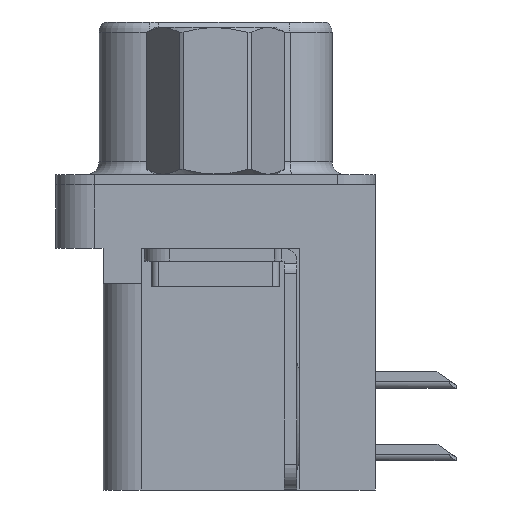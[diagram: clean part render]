
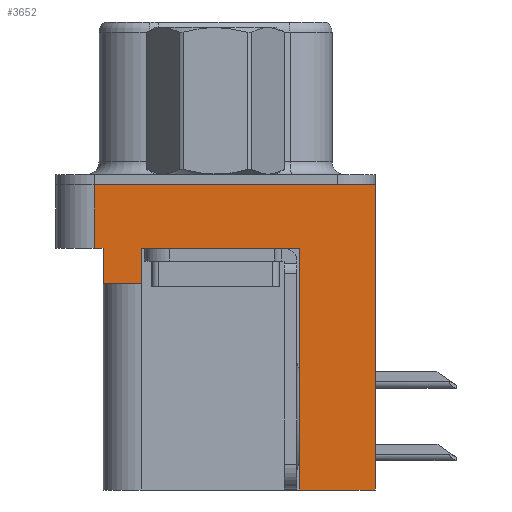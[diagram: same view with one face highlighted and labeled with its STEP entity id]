
A CAD part, left-side view. The second image highlights one B-rep face of the part: STEP entity #3652.
In plain terms, the highlighted planar face has unit normal (-1, 0, 0).
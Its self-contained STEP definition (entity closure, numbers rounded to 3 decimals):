
#145 = VECTOR ( 'NONE', #4610, 1000. ) ;
#225 = EDGE_CURVE ( 'NONE', #10620, #2807, #2601, .T. ) ;
#402 = EDGE_CURVE ( 'NONE', #2580, #18324, #10570, .T. ) ;
#906 = DIRECTION ( 'NONE',  ( 0., -1., 0. ) ) ;
#934 = ORIENTED_EDGE ( 'NONE', *, *, #18183, .T. ) ;
#1684 = DIRECTION ( 'NONE',  ( 0., 1., 0. ) ) ;
#2019 = CARTESIAN_POINT ( 'NONE',  ( -2.91, 2.895, -3.9 ) ) ;
#2459 = ORIENTED_EDGE ( 'NONE', *, *, #12348, .F. ) ;
#2580 = VERTEX_POINT ( 'NONE', #21307 ) ;
#2601 = LINE ( 'NONE', #19234, #7861 ) ;
#2807 = VERTEX_POINT ( 'NONE', #4406 ) ;
#2844 = CARTESIAN_POINT ( 'NONE',  ( -2.91, 2.895, -3.9 ) ) ;
#3044 = CARTESIAN_POINT ( 'NONE',  ( -2.91, 2.895, -2.5 ) ) ;
#3150 = CARTESIAN_POINT ( 'NONE',  ( -2.91, 4.425, -3.9 ) ) ;
#3314 = DIRECTION ( 'NONE',  ( 0., 1., 0. ) ) ;
#3652 = ADVANCED_FACE ( 'NONE', ( #12428 ), #10808, .T. ) ;
#3697 = EDGE_CURVE ( 'NONE', #4193, #3987, #9401, .T. ) ;
#3956 = LINE ( 'NONE', #8661, #17763 ) ;
#3987 = VERTEX_POINT ( 'NONE', #5061 ) ;
#4091 = ORIENTED_EDGE ( 'NONE', *, *, #16174, .F. ) ;
#4193 = VERTEX_POINT ( 'NONE', #5552 ) ;
#4406 = CARTESIAN_POINT ( 'NONE',  ( -2.91, -3.295, -2.5 ) ) ;
#4610 = DIRECTION ( 'NONE',  ( 0., 0., 1. ) ) ;
#5061 = CARTESIAN_POINT ( 'NONE',  ( -2.91, -6.275, 0. ) ) ;
#5238 = VERTEX_POINT ( 'NONE', #3044 ) ;
#5245 = LINE ( 'NONE', #8052, #15231 ) ;
#5309 = VECTOR ( 'NONE', #8683, 1000. ) ;
#5337 = CARTESIAN_POINT ( 'NONE',  ( -2.91, -6.275, -2.5 ) ) ;
#5366 = CARTESIAN_POINT ( 'NONE',  ( -2.91, 4.425, -2.5 ) ) ;
#5552 = CARTESIAN_POINT ( 'NONE',  ( -2.91, -6.275, -12. ) ) ;
#6441 = LINE ( 'NONE', #3150, #13366 ) ;
#7037 = DIRECTION ( 'NONE',  ( 0., 0., 1. ) ) ;
#7841 = VECTOR ( 'NONE', #14482, 1000. ) ;
#7861 = VECTOR ( 'NONE', #10274, 1000. ) ;
#8052 = CARTESIAN_POINT ( 'NONE',  ( -2.91, -6.275, -2.5 ) ) ;
#8111 = EDGE_CURVE ( 'NONE', #14470, #18324, #6441, .T. ) ;
#8661 = CARTESIAN_POINT ( 'NONE',  ( -2.91, -6.275, 0. ) ) ;
#8683 = DIRECTION ( 'NONE',  ( 0., 0., 1. ) ) ;
#8703 = CARTESIAN_POINT ( 'NONE',  ( -2.91, -3.295, -12. ) ) ;
#8809 = CARTESIAN_POINT ( 'NONE',  ( -2.91, -6.275, -2.5 ) ) ;
#9401 = LINE ( 'NONE', #21330, #22953 ) ;
#10274 = DIRECTION ( 'NONE',  ( 0., 0., 1. ) ) ;
#10570 = LINE ( 'NONE', #5337, #7841 ) ;
#10582 = VECTOR ( 'NONE', #1684, 1000. ) ;
#10620 = VERTEX_POINT ( 'NONE', #8703 ) ;
#10808 = PLANE ( 'NONE',  #14883 ) ;
#11205 = EDGE_LOOP ( 'NONE', ( #4091, #13782, #12781, #11669, #22622, #934, #20091, #13751, #2459, #11340 ) ) ;
#11340 = ORIENTED_EDGE ( 'NONE', *, *, #3697, .T. ) ;
#11578 = VECTOR ( 'NONE', #3314, 1000. ) ;
#11669 = ORIENTED_EDGE ( 'NONE', *, *, #8111, .F. ) ;
#12090 = CARTESIAN_POINT ( 'NONE',  ( -2.91, 4.775, -2.5 ) ) ;
#12291 = DIRECTION ( 'NONE',  ( -1., 0., 0. ) ) ;
#12348 = EDGE_CURVE ( 'NONE', #4193, #10620, #18757, .T. ) ;
#12375 = DIRECTION ( 'NONE',  ( 0., 0., 1. ) ) ;
#12428 = FACE_OUTER_BOUND ( 'NONE', #11205, .T. ) ;
#12781 = ORIENTED_EDGE ( 'NONE', *, *, #402, .T. ) ;
#13366 = VECTOR ( 'NONE', #15440, 1000. ) ;
#13526 = CARTESIAN_POINT ( 'NONE',  ( -2.91, -3.295, -12. ) ) ;
#13751 = ORIENTED_EDGE ( 'NONE', *, *, #225, .F. ) ;
#13782 = ORIENTED_EDGE ( 'NONE', *, *, #16688, .F. ) ;
#14445 = VERTEX_POINT ( 'NONE', #2019 ) ;
#14470 = VERTEX_POINT ( 'NONE', #18390 ) ;
#14482 = DIRECTION ( 'NONE',  ( 0., -1., 0. ) ) ;
#14883 = AXIS2_PLACEMENT_3D ( 'NONE', #8809, #12291, #12375 ) ;
#15231 = VECTOR ( 'NONE', #906, 1000. ) ;
#15349 = CARTESIAN_POINT ( 'NONE',  ( -2.91, 4.775, 0. ) ) ;
#15440 = DIRECTION ( 'NONE',  ( 0., 0., 1. ) ) ;
#16174 = EDGE_CURVE ( 'NONE', #21137, #3987, #3956, .T. ) ;
#16688 = EDGE_CURVE ( 'NONE', #2580, #21137, #22472, .T. ) ;
#17763 = VECTOR ( 'NONE', #20867, 1000. ) ;
#18183 = EDGE_CURVE ( 'NONE', #14445, #5238, #22860, .T. ) ;
#18324 = VERTEX_POINT ( 'NONE', #5366 ) ;
#18345 = LINE ( 'NONE', #22970, #10582 ) ;
#18390 = CARTESIAN_POINT ( 'NONE',  ( -2.91, 4.425, -3.9 ) ) ;
#18757 = LINE ( 'NONE', #13526, #11578 ) ;
#19234 = CARTESIAN_POINT ( 'NONE',  ( -2.91, -3.295, -12. ) ) ;
#20091 = ORIENTED_EDGE ( 'NONE', *, *, #22215, .T. ) ;
#20244 = EDGE_CURVE ( 'NONE', #14445, #14470, #18345, .T. ) ;
#20867 = DIRECTION ( 'NONE',  ( 0., -1., 0. ) ) ;
#21137 = VERTEX_POINT ( 'NONE', #15349 ) ;
#21307 = CARTESIAN_POINT ( 'NONE',  ( -2.91, 4.775, -2.5 ) ) ;
#21330 = CARTESIAN_POINT ( 'NONE',  ( -2.91, -6.275, -2.5 ) ) ;
#22215 = EDGE_CURVE ( 'NONE', #5238, #2807, #5245, .T. ) ;
#22472 = LINE ( 'NONE', #12090, #5309 ) ;
#22622 = ORIENTED_EDGE ( 'NONE', *, *, #20244, .F. ) ;
#22860 = LINE ( 'NONE', #2844, #145 ) ;
#22953 = VECTOR ( 'NONE', #7037, 1000. ) ;
#22970 = CARTESIAN_POINT ( 'NONE',  ( -2.91, 4.425, -3.9 ) ) ;
